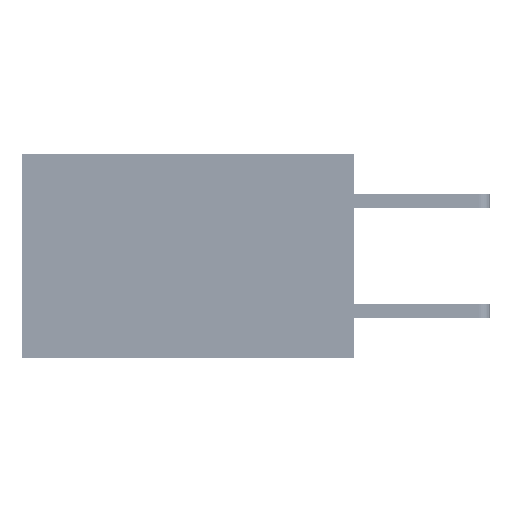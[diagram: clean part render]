
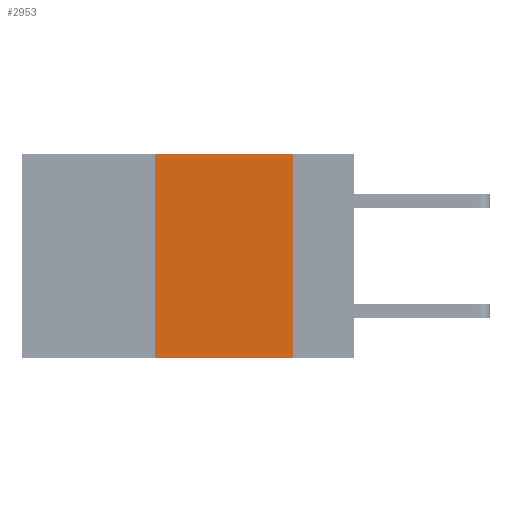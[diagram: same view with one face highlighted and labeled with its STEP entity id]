
A CAD part, left-side view. The second image highlights one B-rep face of the part: STEP entity #2953.
In plain terms, the highlighted planar face has unit normal (-1, 0, 0).
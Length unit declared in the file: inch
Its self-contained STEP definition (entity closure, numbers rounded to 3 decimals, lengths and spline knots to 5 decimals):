
#212 = FACE_OUTER_BOUND ( 'NONE', #10058, .T. ) ;
#1000 = ORIENTED_EDGE ( 'NONE', *, *, #42889, .F. ) ;
#1195 = VERTEX_POINT ( 'NONE', #34686 ) ;
#1974 = LINE ( 'NONE', #29370, #15357 ) ;
#2953 = ADVANCED_FACE ( 'NONE', ( #212 ), #3841, .F. ) ;
#3841 = PLANE ( 'NONE',  #10408 ) ;
#4835 = LINE ( 'NONE', #43336, #28130 ) ;
#4932 = DIRECTION ( 'NONE',  ( 0., -1., 0. ) ) ;
#6917 = ORIENTED_EDGE ( 'NONE', *, *, #24833, .F. ) ;
#7007 = CARTESIAN_POINT ( 'NONE',  ( 0., 0.11, 0. ) ) ;
#10058 = EDGE_LOOP ( 'NONE', ( #6917, #19777, #1000, #31237 ) ) ;
#10228 = VECTOR ( 'NONE', #23970, 39.37008 ) ;
#10408 = AXIS2_PLACEMENT_3D ( 'NONE', #34873, #17432, #10631 ) ;
#10631 = DIRECTION ( 'NONE',  ( 0., 0., -1. ) ) ;
#11534 = CARTESIAN_POINT ( 'NONE',  ( 0., 0.6, 0. ) ) ;
#11626 = DIRECTION ( 'NONE',  ( 0., 0., 1. ) ) ;
#12321 = VERTEX_POINT ( 'NONE', #40498 ) ;
#12998 = VERTEX_POINT ( 'NONE', #19271 ) ;
#15357 = VECTOR ( 'NONE', #4932, 39.37008 ) ;
#17432 = DIRECTION ( 'NONE',  ( 1., 0., 0. ) ) ;
#19271 = CARTESIAN_POINT ( 'NONE',  ( 0., 0.36, 0. ) ) ;
#19777 = ORIENTED_EDGE ( 'NONE', *, *, #30967, .F. ) ;
#23545 = DIRECTION ( 'NONE',  ( 0., 0., -1. ) ) ;
#23970 = DIRECTION ( 'NONE',  ( 0., -1., 0. ) ) ;
#24833 = EDGE_CURVE ( 'NONE', #12321, #1195, #38025, .T. ) ;
#27532 = CARTESIAN_POINT ( 'NONE',  ( 0., 0.36, -0.37 ) ) ;
#28130 = VECTOR ( 'NONE', #11626, 39.37008 ) ;
#28452 = VECTOR ( 'NONE', #23545, 39.37008 ) ;
#29370 = CARTESIAN_POINT ( 'NONE',  ( 0., 0.6, -0.37 ) ) ;
#30967 = EDGE_CURVE ( 'NONE', #12998, #12321, #33041, .T. ) ;
#31237 = ORIENTED_EDGE ( 'NONE', *, *, #33911, .T. ) ;
#33041 = LINE ( 'NONE', #11534, #10228 ) ;
#33911 = EDGE_CURVE ( 'NONE', #39629, #1195, #1974, .T. ) ;
#34686 = CARTESIAN_POINT ( 'NONE',  ( 0., 0.11, -0.37 ) ) ;
#34873 = CARTESIAN_POINT ( 'NONE',  ( 0., 0.6, 0. ) ) ;
#38025 = LINE ( 'NONE', #7007, #28452 ) ;
#39629 = VERTEX_POINT ( 'NONE', #27532 ) ;
#40498 = CARTESIAN_POINT ( 'NONE',  ( 0., 0.11, 0. ) ) ;
#42889 = EDGE_CURVE ( 'NONE', #39629, #12998, #4835, .T. ) ;
#43336 = CARTESIAN_POINT ( 'NONE',  ( 0., 0.36, 0. ) ) ;
